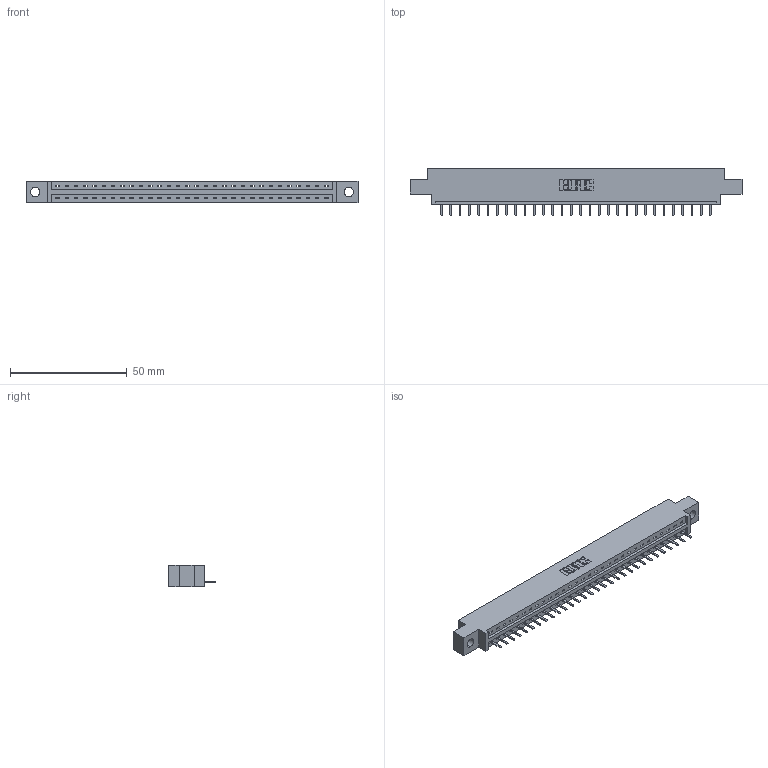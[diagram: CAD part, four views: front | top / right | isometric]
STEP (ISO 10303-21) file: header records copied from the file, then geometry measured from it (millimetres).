
FILE_DESCRIPTION (( 'STEP AP203' ), '1' );
FILE_NAME ('337-030-520-604.STEP', '2019-09-30T23:17:05', ( '' ), ( '' ), 'SwSTEP 2.0', 'SolidWorks 2016', '' );
FILE_SCHEMA (( 'CONFIG_CONTROL_DESIGN' ));
Length unit declared in the file: inch
Products named in the file (3): 345-292-001_345-293-120; 337-030-520-604; 337 Part_0.170 Offset - 0.156 Dia-TH
Assembly tree (31 placements, depth 2):
  337-030-520-604
    337 Part_0.170 Offset - 0.156 Dia-TH
    345-292-001_345-293-120  x30
Bounding box: 141.88 x 20.02 x 9.4 mm (x, y, z)
Volume: 14304.7 mm3; surface area: 14296.2 mm2
Topology: 31 solids, 31 shells, 2098 faces, 6203 edges, 4054 vertices
Faces by surface type: plane 1514, cylinder 584
Entity records: 24101 total; most frequent: CARTESIAN_POINT 4216, ORIENTED_EDGE 4170, DIRECTION 3561, EDGE_CURVE 2085, LINE 1953, VECTOR 1953, VERTEX_POINT 1386, AXIS2_PLACEMENT_3D 804
